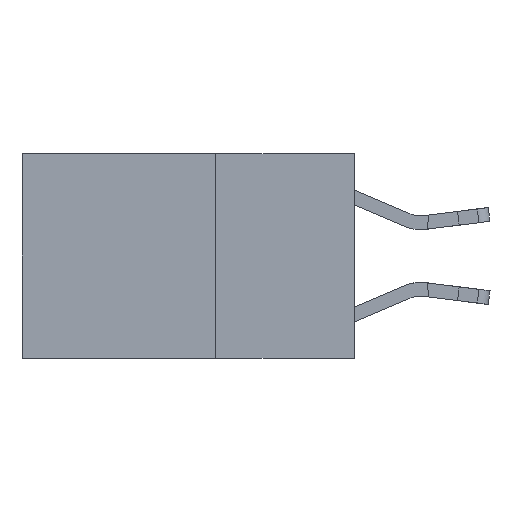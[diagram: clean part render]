
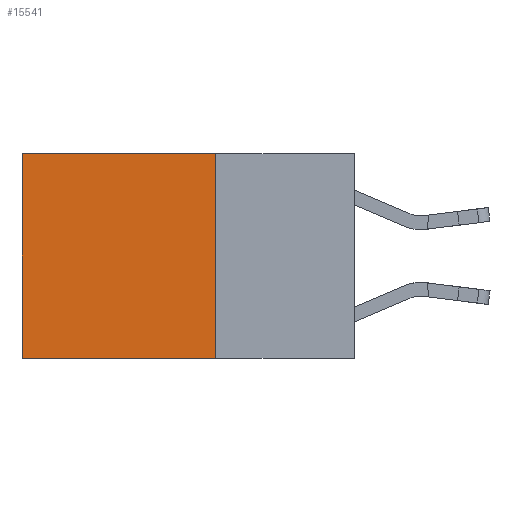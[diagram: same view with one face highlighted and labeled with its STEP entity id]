
A CAD part, left-side view. The second image highlights one B-rep face of the part: STEP entity #15541.
In plain terms, the highlighted planar face has unit normal (-1, 0, 0).
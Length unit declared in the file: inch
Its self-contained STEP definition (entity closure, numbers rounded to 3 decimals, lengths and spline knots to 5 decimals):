
#332 = DIRECTION ( 'NONE',  ( 1., 0., 0. ) ) ;
#816 = EDGE_CURVE ( 'NONE', #9690, #4195, #3935, .T. ) ;
#882 = LINE ( 'NONE', #9721, #1844 ) ;
#1165 = VECTOR ( 'NONE', #9035, 39.37008 ) ;
#1566 = EDGE_CURVE ( 'NONE', #15740, #2906, #7378, .T. ) ;
#1844 = VECTOR ( 'NONE', #14704, 39.37008 ) ;
#1914 = FACE_OUTER_BOUND ( 'NONE', #2075, .T. ) ;
#2075 = EDGE_LOOP ( 'NONE', ( #2682, #3877, #10437, #7615 ) ) ;
#2639 = CARTESIAN_POINT ( 'NONE',  ( 0.2625, 0.6, 0. ) ) ;
#2682 = ORIENTED_EDGE ( 'NONE', *, *, #816, .T. ) ;
#2906 = VERTEX_POINT ( 'NONE', #8401 ) ;
#3877 = ORIENTED_EDGE ( 'NONE', *, *, #5646, .F. ) ;
#3935 = LINE ( 'NONE', #2639, #8721 ) ;
#4195 = VERTEX_POINT ( 'NONE', #7304 ) ;
#5646 = EDGE_CURVE ( 'NONE', #2906, #4195, #882, .T. ) ;
#6937 = PLANE ( 'NONE',  #13365 ) ;
#7304 = CARTESIAN_POINT ( 'NONE',  ( 0.2625, 0.6, -0.37 ) ) ;
#7378 = LINE ( 'NONE', #8559, #9797 ) ;
#7615 = ORIENTED_EDGE ( 'NONE', *, *, #9579, .T. ) ;
#7961 = LINE ( 'NONE', #9123, #1165 ) ;
#8401 = CARTESIAN_POINT ( 'NONE',  ( 0.2625, 0.25, -0.37 ) ) ;
#8559 = CARTESIAN_POINT ( 'NONE',  ( 0.2625, 0.25, 0. ) ) ;
#8721 = VECTOR ( 'NONE', #12694, 39.37008 ) ;
#9013 = CARTESIAN_POINT ( 'NONE',  ( 0.2625, 0.25, 0. ) ) ;
#9035 = DIRECTION ( 'NONE',  ( 0., 1., 0. ) ) ;
#9123 = CARTESIAN_POINT ( 'NONE',  ( 0.2625, 0.25, 0. ) ) ;
#9579 = EDGE_CURVE ( 'NONE', #15740, #9690, #7961, .T. ) ;
#9690 = VERTEX_POINT ( 'NONE', #15819 ) ;
#9721 = CARTESIAN_POINT ( 'NONE',  ( 0.2625, 0.25, -0.37 ) ) ;
#9797 = VECTOR ( 'NONE', #11106, 39.37008 ) ;
#10437 = ORIENTED_EDGE ( 'NONE', *, *, #1566, .F. ) ;
#10588 = CARTESIAN_POINT ( 'NONE',  ( 0.2625, 0.25, 0. ) ) ;
#11106 = DIRECTION ( 'NONE',  ( 0., 0., -1. ) ) ;
#12694 = DIRECTION ( 'NONE',  ( 0., 0., -1. ) ) ;
#12969 = DIRECTION ( 'NONE',  ( 0., 0., -1. ) ) ;
#13365 = AXIS2_PLACEMENT_3D ( 'NONE', #10588, #332, #12969 ) ;
#14704 = DIRECTION ( 'NONE',  ( 0., 1., 0. ) ) ;
#15541 = ADVANCED_FACE ( 'NONE', ( #1914 ), #6937, .F. ) ;
#15740 = VERTEX_POINT ( 'NONE', #9013 ) ;
#15819 = CARTESIAN_POINT ( 'NONE',  ( 0.2625, 0.6, 0. ) ) ;
